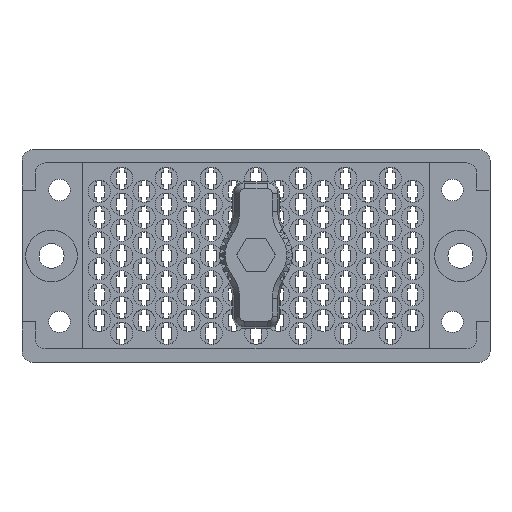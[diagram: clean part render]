
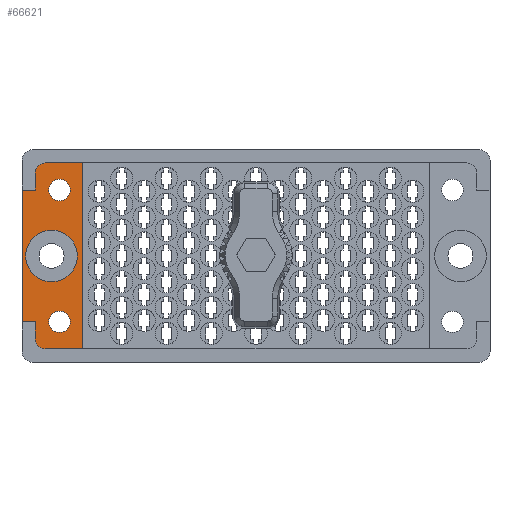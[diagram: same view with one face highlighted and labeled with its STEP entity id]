
A CAD part, top view. The second image highlights one B-rep face of the part: STEP entity #66621.
In plain terms, the highlighted planar face has unit normal (0, 0, 1).
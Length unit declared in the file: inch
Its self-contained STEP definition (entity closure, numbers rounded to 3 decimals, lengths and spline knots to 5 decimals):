
#1538 = FACE_BOUND ( 'NONE', #39665, .T. ) ;
#2160 = CARTESIAN_POINT ( 'NONE',  ( -1.359, 0.617, -0.117 ) ) ;
#3316 = ORIENTED_EDGE ( 'NONE', *, *, #69390, .T. ) ;
#4485 = DIRECTION ( 'NONE',  ( 1., 0., 0. ) ) ;
#4985 = FACE_OUTER_BOUND ( 'NONE', #79049, .T. ) ;
#6160 = DIRECTION ( 'NONE',  ( 1., 0., 0. ) ) ;
#6174 = VERTEX_POINT ( 'NONE', #52709 ) ;
#6504 = AXIS2_PLACEMENT_3D ( 'NONE', #29182, #41512, #4485 ) ;
#6565 = ORIENTED_EDGE ( 'NONE', *, *, #78406, .T. ) ;
#8526 = VERTEX_POINT ( 'NONE', #47765 ) ;
#9538 = VECTOR ( 'NONE', #80008, 39.37008 ) ;
#9740 = ORIENTED_EDGE ( 'NONE', *, *, #48296, .T. ) ;
#10347 = LINE ( 'NONE', #15336, #76108 ) ;
#10350 = VERTEX_POINT ( 'NONE', #59235 ) ;
#10661 = CARTESIAN_POINT ( 'NONE',  ( -1.005, -0.54, -0.117 ) ) ;
#10740 = VECTOR ( 'NONE', #12204, 39.37008 ) ;
#12204 = DIRECTION ( 'NONE',  ( -1., 0., 0. ) ) ;
#12851 = AXIS2_PLACEMENT_3D ( 'NONE', #79856, #73180, #66841 ) ;
#13208 = ORIENTED_EDGE ( 'NONE', *, *, #71085, .F. ) ;
#13230 = CARTESIAN_POINT ( 'NONE',  ( -1.2205, -0.478, -0.117 ) ) ;
#13535 = CIRCLE ( 'NONE', #6504, 0.0625 ) ;
#14721 = DIRECTION ( 'NONE',  ( 1., 0., 0. ) ) ;
#15336 = CARTESIAN_POINT ( 'NONE',  ( -1.2825, 0., -0.117 ) ) ;
#16025 = VERTEX_POINT ( 'NONE', #42655 ) ;
#16154 = DIRECTION ( 'NONE',  ( 0., -1., 0. ) ) ;
#16543 = LINE ( 'NONE', #51483, #23338 ) ;
#16638 = VECTOR ( 'NONE', #52418, 39.37008 ) ;
#16963 = CIRCLE ( 'NONE', #32386, 0.062 ) ;
#17849 = EDGE_CURVE ( 'NONE', #10350, #66787, #69670, .T. ) ;
#18799 = CARTESIAN_POINT ( 'NONE',  ( 0., -0.3825, -0.117 ) ) ;
#18822 = CARTESIAN_POINT ( 'NONE',  ( 0., 0.3825, -0.117 ) ) ;
#19542 = LINE ( 'NONE', #48630, #71571 ) ;
#19650 = CARTESIAN_POINT ( 'NONE',  ( -1.141, -0.3825, -0.117 ) ) ;
#19768 = ORIENTED_EDGE ( 'NONE', *, *, #57090, .T. ) ;
#20052 = VERTEX_POINT ( 'NONE', #32193 ) ;
#20093 = EDGE_CURVE ( 'NONE', #26403, #6174, #36496, .T. ) ;
#20438 = CARTESIAN_POINT ( 'NONE',  ( -1.0375, 0., -0.117 ) ) ;
#21150 = ORIENTED_EDGE ( 'NONE', *, *, #22328, .F. ) ;
#21455 = EDGE_CURVE ( 'NONE', #79439, #20052, #63784, .T. ) ;
#22068 = EDGE_CURVE ( 'NONE', #23487, #51452, #16543, .T. ) ;
#22328 = EDGE_CURVE ( 'NONE', #20052, #79439, #13535, .T. ) ;
#22671 = VECTOR ( 'NONE', #26603, 39.37008 ) ;
#23338 = VECTOR ( 'NONE', #70130, 39.37008 ) ;
#23449 = VERTEX_POINT ( 'NONE', #47954 ) ;
#23487 = VERTEX_POINT ( 'NONE', #10661 ) ;
#25056 = VECTOR ( 'NONE', #81407, 39.37008 ) ;
#25413 = CIRCLE ( 'NONE', #69865, 0.0625 ) ;
#25439 = CIRCLE ( 'NONE', #77777, 0.15 ) ;
#25753 = CARTESIAN_POINT ( 'NONE',  ( -1.1875, 0., -0.117 ) ) ;
#26355 = ORIENTED_EDGE ( 'NONE', *, *, #57466, .T. ) ;
#26362 = DIRECTION ( 'NONE',  ( 1., 0., 0. ) ) ;
#26403 = VERTEX_POINT ( 'NONE', #37134 ) ;
#26603 = DIRECTION ( 'NONE',  ( -1., 0., 0. ) ) ;
#27418 = CARTESIAN_POINT ( 'NONE',  ( 0., 0.54, -0.117 ) ) ;
#27749 = DIRECTION ( 'NONE',  ( 1., 0., 0. ) ) ;
#27773 = CARTESIAN_POINT ( 'NONE',  ( -1.141, -0.3825, -0.117 ) ) ;
#28207 = EDGE_LOOP ( 'NONE', ( #21150, #56115 ) ) ;
#28974 = PLANE ( 'NONE',  #12851 ) ;
#29005 = ORIENTED_EDGE ( 'NONE', *, *, #41502, .T. ) ;
#29182 = CARTESIAN_POINT ( 'NONE',  ( -1.141, 0.3825, -0.117 ) ) ;
#29249 = CARTESIAN_POINT ( 'NONE',  ( -1.2205, 0.478, -0.117 ) ) ;
#31519 = ORIENTED_EDGE ( 'NONE', *, *, #59020, .T. ) ;
#31927 = DIRECTION ( 'NONE',  ( 0., 0., 1. ) ) ;
#32193 = CARTESIAN_POINT ( 'NONE',  ( -1.2035, 0.3825, -0.117 ) ) ;
#32323 = LINE ( 'NONE', #2160, #16638 ) ;
#32386 = AXIS2_PLACEMENT_3D ( 'NONE', #29249, #73197, #48190 ) ;
#33246 = CARTESIAN_POINT ( 'NONE',  ( -1.141, 0.3825, -0.117 ) ) ;
#33516 = DIRECTION ( 'NONE',  ( 0., 0., 1. ) ) ;
#36496 = CIRCLE ( 'NONE', #51562, 0.0625 ) ;
#36863 = CARTESIAN_POINT ( 'NONE',  ( -1.2205, -0.54, -0.117 ) ) ;
#37134 = CARTESIAN_POINT ( 'NONE',  ( -1.0785, -0.3825, -0.117 ) ) ;
#37493 = ORIENTED_EDGE ( 'NONE', *, *, #47280, .T. ) ;
#38732 = LINE ( 'NONE', #18799, #25056 ) ;
#39665 = EDGE_LOOP ( 'NONE', ( #13208, #72459 ) ) ;
#39689 = VERTEX_POINT ( 'NONE', #41935 ) ;
#40363 = DIRECTION ( 'NONE',  ( 0., 0., 1. ) ) ;
#40807 = VERTEX_POINT ( 'NONE', #71650 ) ;
#41502 = EDGE_CURVE ( 'NONE', #39689, #51452, #43704, .T. ) ;
#41512 = DIRECTION ( 'NONE',  ( 0., 0., 1. ) ) ;
#41935 = CARTESIAN_POINT ( 'NONE',  ( -1.2825, -0.478, -0.117 ) ) ;
#42655 = CARTESIAN_POINT ( 'NONE',  ( -1.359, -0.3825, -0.117 ) ) ;
#43704 = CIRCLE ( 'NONE', #76027, 0.062 ) ;
#45263 = EDGE_CURVE ( 'NONE', #6174, #26403, #25413, .T. ) ;
#46049 = LINE ( 'NONE', #18822, #10740 ) ;
#47280 = EDGE_CURVE ( 'NONE', #65803, #78339, #69860, .T. ) ;
#47765 = CARTESIAN_POINT ( 'NONE',  ( -1.2825, 0.478, -0.117 ) ) ;
#47954 = CARTESIAN_POINT ( 'NONE',  ( -1.2825, -0.3825, -0.117 ) ) ;
#48190 = DIRECTION ( 'NONE',  ( 1., 0., 0. ) ) ;
#48296 = EDGE_CURVE ( 'NONE', #40807, #79898, #46049, .T. ) ;
#48630 = CARTESIAN_POINT ( 'NONE',  ( -1.005, 0.617, -0.117 ) ) ;
#49468 = FACE_BOUND ( 'NONE', #28207, .T. ) ;
#51452 = VERTEX_POINT ( 'NONE', #36863 ) ;
#51483 = CARTESIAN_POINT ( 'NONE',  ( 0., -0.54, -0.117 ) ) ;
#51562 = AXIS2_PLACEMENT_3D ( 'NONE', #27773, #40363, #78070 ) ;
#52298 = DIRECTION ( 'NONE',  ( 0., 0., 1. ) ) ;
#52418 = DIRECTION ( 'NONE',  ( 0., -1., 0. ) ) ;
#52709 = CARTESIAN_POINT ( 'NONE',  ( -1.2035, -0.3825, -0.117 ) ) ;
#53316 = EDGE_CURVE ( 'NONE', #23449, #16025, #38732, .T. ) ;
#54119 = CARTESIAN_POINT ( 'NONE',  ( -1.2825, 0., -0.117 ) ) ;
#54171 = ORIENTED_EDGE ( 'NONE', *, *, #20093, .F. ) ;
#54960 = DIRECTION ( 'NONE',  ( 0., 1., 0. ) ) ;
#55670 = LINE ( 'NONE', #54119, #9538 ) ;
#56115 = ORIENTED_EDGE ( 'NONE', *, *, #21455, .F. ) ;
#56727 = AXIS2_PLACEMENT_3D ( 'NONE', #78137, #52298, #14721 ) ;
#57090 = EDGE_CURVE ( 'NONE', #23487, #65803, #19542, .T. ) ;
#57114 = CARTESIAN_POINT ( 'NONE',  ( -1.005, 0.54, -0.117 ) ) ;
#57413 = CARTESIAN_POINT ( 'NONE',  ( -1.2205, 0.54, -0.117 ) ) ;
#57466 = EDGE_CURVE ( 'NONE', #79898, #16025, #32323, .T. ) ;
#59020 = EDGE_CURVE ( 'NONE', #23449, #39689, #55670, .T. ) ;
#59235 = CARTESIAN_POINT ( 'NONE',  ( -1.3375, 0., -0.117 ) ) ;
#59999 = CARTESIAN_POINT ( 'NONE',  ( -1.359, 0.3825, -0.117 ) ) ;
#61955 = ORIENTED_EDGE ( 'NONE', *, *, #45263, .F. ) ;
#63647 = DIRECTION ( 'NONE',  ( 1., 0., 0. ) ) ;
#63752 = FACE_BOUND ( 'NONE', #65924, .T. ) ;
#63784 = CIRCLE ( 'NONE', #70568, 0.0625 ) ;
#65803 = VERTEX_POINT ( 'NONE', #57114 ) ;
#65924 = EDGE_LOOP ( 'NONE', ( #61955, #54171 ) ) ;
#66621 = ADVANCED_FACE ( 'NONE', ( #63752, #49468, #1538, #4985 ), #28974, .T. ) ;
#66787 = VERTEX_POINT ( 'NONE', #20438 ) ;
#66841 = DIRECTION ( 'NONE',  ( 1., 0., 0. ) ) ;
#69234 = DIRECTION ( 'NONE',  ( 0., 0., 1. ) ) ;
#69390 = EDGE_CURVE ( 'NONE', #78339, #8526, #16963, .T. ) ;
#69670 = CIRCLE ( 'NONE', #56727, 0.15 ) ;
#69860 = LINE ( 'NONE', #27418, #22671 ) ;
#69865 = AXIS2_PLACEMENT_3D ( 'NONE', #19650, #31927, #6160 ) ;
#70130 = DIRECTION ( 'NONE',  ( -1., 0., 0. ) ) ;
#70568 = AXIS2_PLACEMENT_3D ( 'NONE', #33246, #33516, #27749 ) ;
#71085 = EDGE_CURVE ( 'NONE', #66787, #10350, #25439, .T. ) ;
#71571 = VECTOR ( 'NONE', #54960, 39.37008 ) ;
#71650 = CARTESIAN_POINT ( 'NONE',  ( -1.2825, 0.3825, -0.117 ) ) ;
#72459 = ORIENTED_EDGE ( 'NONE', *, *, #17849, .F. ) ;
#73180 = DIRECTION ( 'NONE',  ( 0., 0., 1. ) ) ;
#73197 = DIRECTION ( 'NONE',  ( 0., 0., 1. ) ) ;
#75741 = DIRECTION ( 'NONE',  ( 0., 0., 1. ) ) ;
#76027 = AXIS2_PLACEMENT_3D ( 'NONE', #13230, #69234, #26362 ) ;
#76108 = VECTOR ( 'NONE', #16154, 39.37008 ) ;
#76578 = ORIENTED_EDGE ( 'NONE', *, *, #22068, .F. ) ;
#76708 = CARTESIAN_POINT ( 'NONE',  ( -1.0785, 0.3825, -0.117 ) ) ;
#77777 = AXIS2_PLACEMENT_3D ( 'NONE', #25753, #75741, #63647 ) ;
#78070 = DIRECTION ( 'NONE',  ( 1., 0., 0. ) ) ;
#78137 = CARTESIAN_POINT ( 'NONE',  ( -1.1875, 0., -0.117 ) ) ;
#78339 = VERTEX_POINT ( 'NONE', #57413 ) ;
#78406 = EDGE_CURVE ( 'NONE', #8526, #40807, #10347, .T. ) ;
#79049 = EDGE_LOOP ( 'NONE', ( #31519, #29005, #76578, #19768, #37493, #3316, #6565, #9740, #26355, #79963 ) ) ;
#79439 = VERTEX_POINT ( 'NONE', #76708 ) ;
#79856 = CARTESIAN_POINT ( 'NONE',  ( -1.359, -0.617, -0.117 ) ) ;
#79898 = VERTEX_POINT ( 'NONE', #59999 ) ;
#79963 = ORIENTED_EDGE ( 'NONE', *, *, #53316, .F. ) ;
#80008 = DIRECTION ( 'NONE',  ( 0., -1., 0. ) ) ;
#81407 = DIRECTION ( 'NONE',  ( -1., 0., 0. ) ) ;
